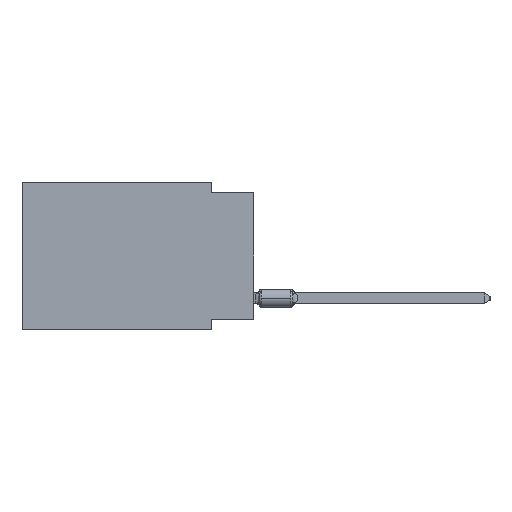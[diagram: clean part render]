
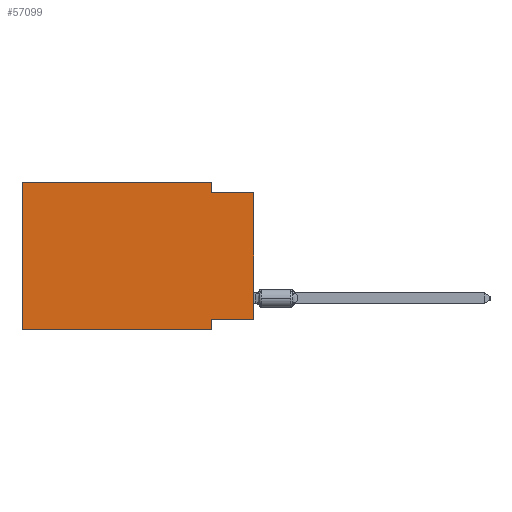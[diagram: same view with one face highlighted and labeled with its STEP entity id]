
A CAD part, left-side view. The second image highlights one B-rep face of the part: STEP entity #57099.
In plain terms, the highlighted planar face has unit normal (-1, 0, 0).
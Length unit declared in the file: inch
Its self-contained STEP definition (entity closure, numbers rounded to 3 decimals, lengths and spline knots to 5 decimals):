
#183 = VECTOR ( 'NONE', #18136, 39.37008 ) ;
#302 = DIRECTION ( 'NONE',  ( 0., -1., 0. ) ) ;
#1445 = VERTEX_POINT ( 'NONE', #36432 ) ;
#4224 = CARTESIAN_POINT ( 'NONE',  ( 0., 0., -0.025 ) ) ;
#5759 = EDGE_CURVE ( 'NONE', #43603, #55293, #53491, .T. ) ;
#7384 = LINE ( 'NONE', #57271, #47512 ) ;
#7629 = LINE ( 'NONE', #34104, #25946 ) ;
#7954 = VERTEX_POINT ( 'NONE', #41816 ) ;
#8020 = EDGE_CURVE ( 'NONE', #26565, #39335, #7629, .T. ) ;
#8623 = CARTESIAN_POINT ( 'NONE',  ( 0., 0.55, -0.35 ) ) ;
#11001 = CARTESIAN_POINT ( 'NONE',  ( 0., 0.1, -0.35 ) ) ;
#12233 = CARTESIAN_POINT ( 'NONE',  ( 0., 0.1, -0.325 ) ) ;
#12587 = VECTOR ( 'NONE', #302, 39.37008 ) ;
#13083 = VECTOR ( 'NONE', #41822, 39.37008 ) ;
#13390 = LINE ( 'NONE', #58533, #183 ) ;
#13718 = DIRECTION ( 'NONE',  ( 0., -1., 0. ) ) ;
#13807 = CARTESIAN_POINT ( 'NONE',  ( 0., 0.55, -0.35 ) ) ;
#14495 = LINE ( 'NONE', #28184, #13083 ) ;
#16370 = EDGE_CURVE ( 'NONE', #19068, #55293, #34302, .T. ) ;
#17611 = VECTOR ( 'NONE', #38462, 39.37008 ) ;
#18033 = EDGE_CURVE ( 'NONE', #1445, #19068, #13390, .T. ) ;
#18136 = DIRECTION ( 'NONE',  ( 0., 1., 0. ) ) ;
#19068 = VERTEX_POINT ( 'NONE', #12233 ) ;
#21619 = ORIENTED_EDGE ( 'NONE', *, *, #41868, .F. ) ;
#22851 = VECTOR ( 'NONE', #58027, 39.37008 ) ;
#23549 = CARTESIAN_POINT ( 'NONE',  ( 0., 0.55, 0. ) ) ;
#23564 = PLANE ( 'NONE',  #41913 ) ;
#25946 = VECTOR ( 'NONE', #30525, 39.37008 ) ;
#26565 = VERTEX_POINT ( 'NONE', #23549 ) ;
#28019 = CARTESIAN_POINT ( 'NONE',  ( 0., 0.55, 0. ) ) ;
#28184 = CARTESIAN_POINT ( 'NONE',  ( 0., 0.55, 0. ) ) ;
#29850 = EDGE_CURVE ( 'NONE', #1445, #35077, #7384, .T. ) ;
#30173 = CARTESIAN_POINT ( 'NONE',  ( 0., 0.1, 0. ) ) ;
#30525 = DIRECTION ( 'NONE',  ( 0., -1., 0. ) ) ;
#32467 = FACE_OUTER_BOUND ( 'NONE', #42062, .T. ) ;
#33841 = ORIENTED_EDGE ( 'NONE', *, *, #8020, .F. ) ;
#34104 = CARTESIAN_POINT ( 'NONE',  ( 0., 0.55, 0. ) ) ;
#34302 = LINE ( 'NONE', #47357, #17611 ) ;
#34715 = CARTESIAN_POINT ( 'NONE',  ( 0., 0., -0.025 ) ) ;
#34803 = ORIENTED_EDGE ( 'NONE', *, *, #16370, .F. ) ;
#34907 = LINE ( 'NONE', #30173, #22851 ) ;
#35077 = VERTEX_POINT ( 'NONE', #34715 ) ;
#36432 = CARTESIAN_POINT ( 'NONE',  ( 0., 0., -0.325 ) ) ;
#38462 = DIRECTION ( 'NONE',  ( 0., 0., -1. ) ) ;
#39335 = VERTEX_POINT ( 'NONE', #40633 ) ;
#39534 = ORIENTED_EDGE ( 'NONE', *, *, #56403, .F. ) ;
#39773 = ORIENTED_EDGE ( 'NONE', *, *, #5759, .T. ) ;
#40633 = CARTESIAN_POINT ( 'NONE',  ( 0., 0.1, 0. ) ) ;
#40756 = LINE ( 'NONE', #4224, #50453 ) ;
#41347 = ORIENTED_EDGE ( 'NONE', *, *, #54716, .F. ) ;
#41816 = CARTESIAN_POINT ( 'NONE',  ( 0., 0.1, -0.025 ) ) ;
#41822 = DIRECTION ( 'NONE',  ( 0., 0., 1. ) ) ;
#41868 = EDGE_CURVE ( 'NONE', #43603, #26565, #14495, .T. ) ;
#41913 = AXIS2_PLACEMENT_3D ( 'NONE', #28019, #42565, #56194 ) ;
#42062 = EDGE_LOOP ( 'NONE', ( #43791, #39534, #41347, #33841, #21619, #39773, #34803, #56882 ) ) ;
#42565 = DIRECTION ( 'NONE',  ( 1., 0., 0. ) ) ;
#43603 = VERTEX_POINT ( 'NONE', #13807 ) ;
#43791 = ORIENTED_EDGE ( 'NONE', *, *, #29850, .T. ) ;
#47357 = CARTESIAN_POINT ( 'NONE',  ( 0., 0.1, -0.35 ) ) ;
#47512 = VECTOR ( 'NONE', #48078, 39.37008 ) ;
#48078 = DIRECTION ( 'NONE',  ( 0., 0., 1. ) ) ;
#50453 = VECTOR ( 'NONE', #13718, 39.37008 ) ;
#53491 = LINE ( 'NONE', #8623, #12587 ) ;
#54716 = EDGE_CURVE ( 'NONE', #39335, #7954, #34907, .T. ) ;
#55293 = VERTEX_POINT ( 'NONE', #11001 ) ;
#56194 = DIRECTION ( 'NONE',  ( 0., 0., -1. ) ) ;
#56403 = EDGE_CURVE ( 'NONE', #7954, #35077, #40756, .T. ) ;
#56882 = ORIENTED_EDGE ( 'NONE', *, *, #18033, .F. ) ;
#57099 = ADVANCED_FACE ( 'NONE', ( #32467 ), #23564, .F. ) ;
#57271 = CARTESIAN_POINT ( 'NONE',  ( 0., 0., 0. ) ) ;
#58027 = DIRECTION ( 'NONE',  ( 0., 0., -1. ) ) ;
#58533 = CARTESIAN_POINT ( 'NONE',  ( 0., 0., -0.325 ) ) ;
